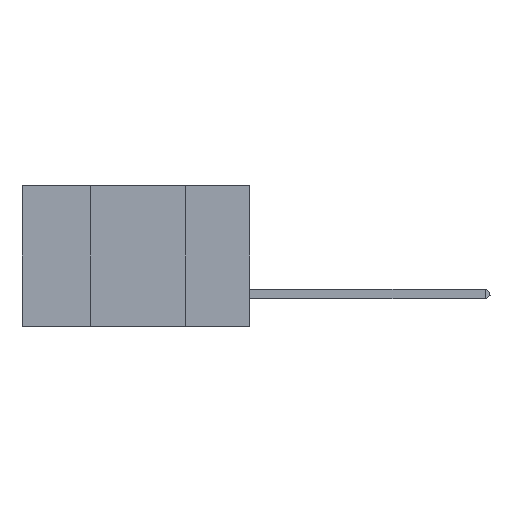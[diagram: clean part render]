
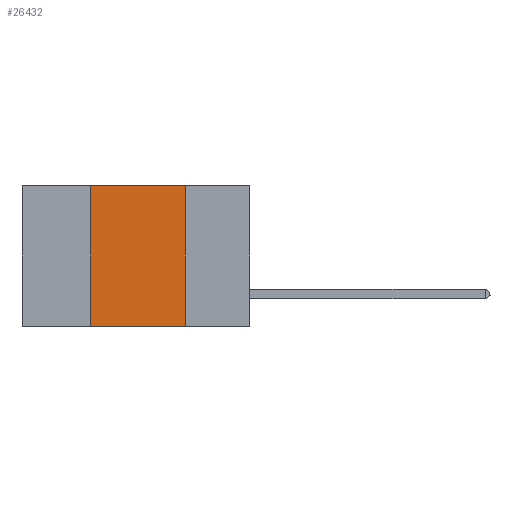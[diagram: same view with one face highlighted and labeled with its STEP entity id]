
A CAD part, left-side view. The second image highlights one B-rep face of the part: STEP entity #26432.
In plain terms, the highlighted planar face has unit normal (-1, 0, 0).
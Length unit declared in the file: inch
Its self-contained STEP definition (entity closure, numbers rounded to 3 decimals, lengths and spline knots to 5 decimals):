
#1097 = EDGE_CURVE ( 'NONE', #33469, #14508, #5694, .T. ) ;
#3540 = EDGE_CURVE ( 'NONE', #33469, #25615, #19072, .T. ) ;
#4700 = CARTESIAN_POINT ( 'NONE',  ( 0., 0.6, -0.37 ) ) ;
#4809 = CARTESIAN_POINT ( 'NONE',  ( 0., 0.17, -0.37 ) ) ;
#5694 = LINE ( 'NONE', #35249, #40565 ) ;
#6754 = CARTESIAN_POINT ( 'NONE',  ( 0., 0.42, -0.37 ) ) ;
#6909 = EDGE_CURVE ( 'NONE', #14508, #14846, #46413, .T. ) ;
#6982 = VECTOR ( 'NONE', #9120, 39.37008 ) ;
#9120 = DIRECTION ( 'NONE',  ( 0., -1., 0. ) ) ;
#9348 = ORIENTED_EDGE ( 'NONE', *, *, #1097, .F. ) ;
#11434 = DIRECTION ( 'NONE',  ( 1., 0., 0. ) ) ;
#14508 = VERTEX_POINT ( 'NONE', #19900 ) ;
#14635 = PLANE ( 'NONE',  #45150 ) ;
#14671 = CARTESIAN_POINT ( 'NONE',  ( 0., 0.6, 0. ) ) ;
#14846 = VERTEX_POINT ( 'NONE', #16239 ) ;
#14901 = CARTESIAN_POINT ( 'NONE',  ( 0., 0.6, 0. ) ) ;
#15047 = VECTOR ( 'NONE', #24635, 39.37008 ) ;
#16069 = EDGE_CURVE ( 'NONE', #14846, #25615, #24690, .T. ) ;
#16239 = CARTESIAN_POINT ( 'NONE',  ( 0., 0.17, 0. ) ) ;
#19072 = LINE ( 'NONE', #4700, #39885 ) ;
#19900 = CARTESIAN_POINT ( 'NONE',  ( 0., 0.42, 0. ) ) ;
#21192 = EDGE_LOOP ( 'NONE', ( #21405, #31496, #9348, #35499 ) ) ;
#21405 = ORIENTED_EDGE ( 'NONE', *, *, #16069, .F. ) ;
#21455 = CARTESIAN_POINT ( 'NONE',  ( 0., 0.17, 0. ) ) ;
#24635 = DIRECTION ( 'NONE',  ( 0., 0., -1. ) ) ;
#24690 = LINE ( 'NONE', #21455, #15047 ) ;
#25615 = VERTEX_POINT ( 'NONE', #4809 ) ;
#26432 = ADVANCED_FACE ( 'NONE', ( #33759 ), #14635, .F. ) ;
#29930 = DIRECTION ( 'NONE',  ( 0., -1., 0. ) ) ;
#31496 = ORIENTED_EDGE ( 'NONE', *, *, #6909, .F. ) ;
#33469 = VERTEX_POINT ( 'NONE', #6754 ) ;
#33759 = FACE_OUTER_BOUND ( 'NONE', #21192, .T. ) ;
#35249 = CARTESIAN_POINT ( 'NONE',  ( 0., 0.42, 0. ) ) ;
#35499 = ORIENTED_EDGE ( 'NONE', *, *, #3540, .T. ) ;
#36891 = DIRECTION ( 'NONE',  ( 0., 0., -1. ) ) ;
#38586 = DIRECTION ( 'NONE',  ( 0., 0., 1. ) ) ;
#39885 = VECTOR ( 'NONE', #29930, 39.37008 ) ;
#40565 = VECTOR ( 'NONE', #38586, 39.37008 ) ;
#45150 = AXIS2_PLACEMENT_3D ( 'NONE', #14901, #11434, #36891 ) ;
#46413 = LINE ( 'NONE', #14671, #6982 ) ;
